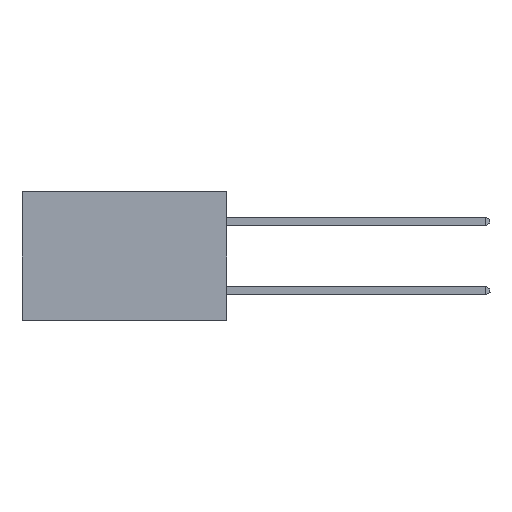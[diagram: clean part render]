
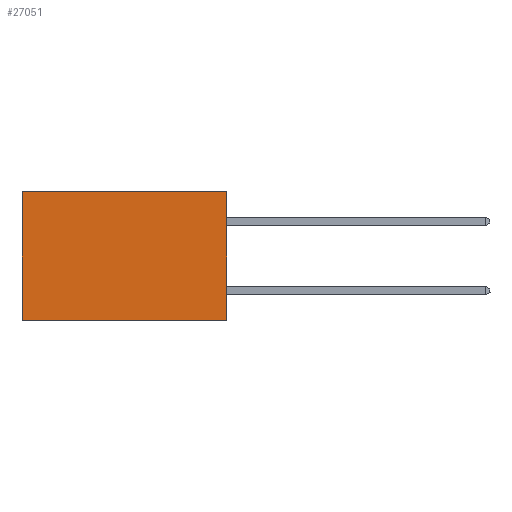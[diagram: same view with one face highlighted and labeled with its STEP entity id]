
A CAD part, left-side view. The second image highlights one B-rep face of the part: STEP entity #27051.
In plain terms, the highlighted planar face has unit normal (-1, 0, 0).
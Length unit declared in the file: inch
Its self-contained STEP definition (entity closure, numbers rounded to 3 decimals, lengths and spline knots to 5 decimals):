
#202 = DIRECTION ( 'NONE',  ( 0., 0., -1. ) ) ;
#1041 = EDGE_CURVE ( 'NONE', #26897, #8974, #10115, .T. ) ;
#1943 = CARTESIAN_POINT ( 'NONE',  ( 0.277, 0.59, -0.37 ) ) ;
#2315 = CARTESIAN_POINT ( 'NONE',  ( 0.277, 0.59, -0.37 ) ) ;
#2912 = VECTOR ( 'NONE', #202, 39.37008 ) ;
#3894 = VECTOR ( 'NONE', #20340, 39.37008 ) ;
#4056 = CARTESIAN_POINT ( 'NONE',  ( 0.277, 0., -0.37 ) ) ;
#4583 = LINE ( 'NONE', #26789, #3894 ) ;
#5060 = FACE_OUTER_BOUND ( 'NONE', #10311, .T. ) ;
#6723 = VERTEX_POINT ( 'NONE', #11401 ) ;
#7270 = ORIENTED_EDGE ( 'NONE', *, *, #18817, .F. ) ;
#7540 = PLANE ( 'NONE',  #22116 ) ;
#7838 = EDGE_CURVE ( 'NONE', #26177, #26897, #4583, .T. ) ;
#7923 = VECTOR ( 'NONE', #19306, 39.37008 ) ;
#8974 = VERTEX_POINT ( 'NONE', #1943 ) ;
#9739 = DIRECTION ( 'NONE',  ( 1., 0., 0. ) ) ;
#10115 = LINE ( 'NONE', #2315, #2912 ) ;
#10144 = VECTOR ( 'NONE', #16045, 39.37008 ) ;
#10311 = EDGE_LOOP ( 'NONE', ( #11746, #7270, #19691, #19804 ) ) ;
#10814 = LINE ( 'NONE', #26888, #10144 ) ;
#11401 = CARTESIAN_POINT ( 'NONE',  ( 0.277, 0., -0.37 ) ) ;
#11728 = CARTESIAN_POINT ( 'NONE',  ( 0.277, 0., 0. ) ) ;
#11746 = ORIENTED_EDGE ( 'NONE', *, *, #1041, .T. ) ;
#15680 = EDGE_CURVE ( 'NONE', #26177, #6723, #25286, .T. ) ;
#16045 = DIRECTION ( 'NONE',  ( 0., 1., 0. ) ) ;
#18817 = EDGE_CURVE ( 'NONE', #6723, #8974, #10814, .T. ) ;
#19306 = DIRECTION ( 'NONE',  ( 0., 0., -1. ) ) ;
#19691 = ORIENTED_EDGE ( 'NONE', *, *, #15680, .F. ) ;
#19804 = ORIENTED_EDGE ( 'NONE', *, *, #7838, .T. ) ;
#20340 = DIRECTION ( 'NONE',  ( 0., 1., 0. ) ) ;
#20591 = CARTESIAN_POINT ( 'NONE',  ( 0.277, 0., -0.37 ) ) ;
#22116 = AXIS2_PLACEMENT_3D ( 'NONE', #20591, #9739, #24963 ) ;
#24963 = DIRECTION ( 'NONE',  ( 0., 0., -1. ) ) ;
#25203 = CARTESIAN_POINT ( 'NONE',  ( 0.277, 0.59, 0. ) ) ;
#25286 = LINE ( 'NONE', #4056, #7923 ) ;
#26177 = VERTEX_POINT ( 'NONE', #11728 ) ;
#26789 = CARTESIAN_POINT ( 'NONE',  ( 0.277, 0., 0. ) ) ;
#26888 = CARTESIAN_POINT ( 'NONE',  ( 0.277, 0., -0.37 ) ) ;
#26897 = VERTEX_POINT ( 'NONE', #25203 ) ;
#27051 = ADVANCED_FACE ( 'NONE', ( #5060 ), #7540, .F. ) ;
